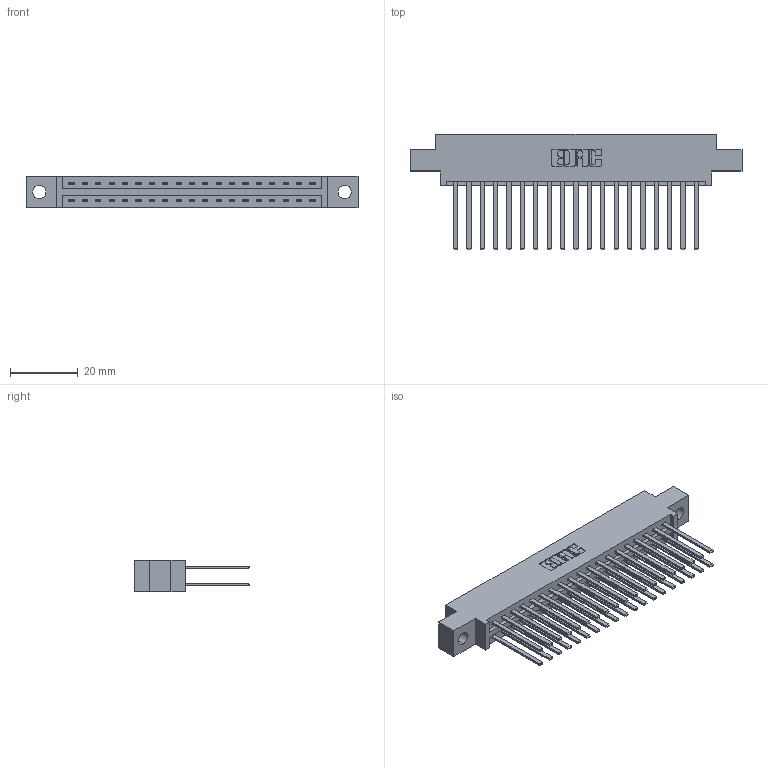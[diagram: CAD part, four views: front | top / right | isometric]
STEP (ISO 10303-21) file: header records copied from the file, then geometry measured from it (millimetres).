
FILE_DESCRIPTION (( 'STEP AP203' ), '1' );
FILE_NAME ('387-038-544-804.STEP', '2018-09-19T06:05:39', ( '' ), ( '' ), 'SwSTEP 2.0', 'SolidWorks 2016', '' );
FILE_SCHEMA (( 'CONFIG_CONTROL_DESIGN' ));
Length unit declared in the file: inch
Products named in the file (3): 337 Part_0.170 Offset - 0.156 Dia-TH; 345-292-001_345-293-144; 387-038-544-804
Assembly tree (39 placements, depth 2):
  387-038-544-804
    337 Part_0.170 Offset - 0.156 Dia-TH
    345-292-001_345-293-144  x38
Bounding box: 98.3 x 34.3 x 9.4 mm (x, y, z)
Volume: 10380.6 mm3; surface area: 13157.3 mm2
Topology: 39 solids, 39 shells, 1942 faces, 5757 edges, 3786 vertices
Faces by surface type: plane 1366, cylinder 576
Entity records: 17657 total; most frequent: CARTESIAN_POINT 2994, ORIENTED_EDGE 2930, DIRECTION 2585, EDGE_CURVE 1465, VECTOR 1341, LINE 1341, VERTEX_POINT 974, AXIS2_PLACEMENT_3D 622
